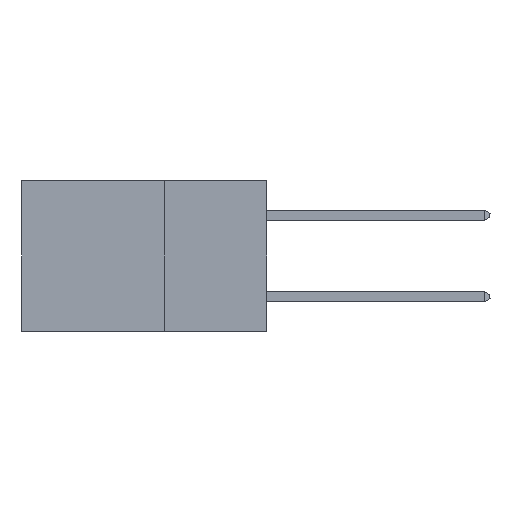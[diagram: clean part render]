
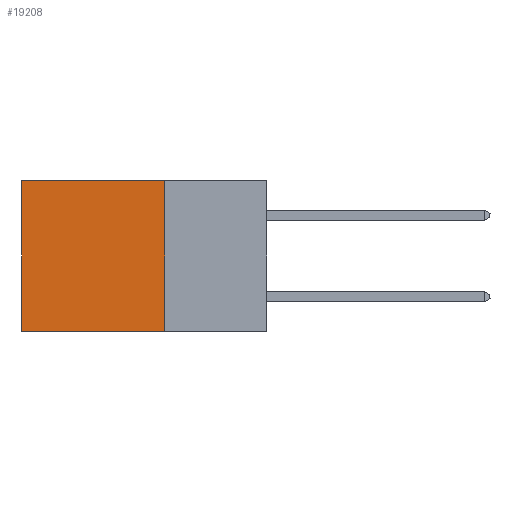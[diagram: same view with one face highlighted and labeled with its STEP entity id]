
A CAD part, left-side view. The second image highlights one B-rep face of the part: STEP entity #19208.
In plain terms, the highlighted planar face has unit normal (-1, 0, 0).
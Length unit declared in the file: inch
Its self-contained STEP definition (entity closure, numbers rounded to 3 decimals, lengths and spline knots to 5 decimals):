
#110 = LINE ( 'NONE', #9441, #12483 ) ;
#734 = VERTEX_POINT ( 'NONE', #19509 ) ;
#827 = CARTESIAN_POINT ( 'NONE',  ( 0.2875, 0.25, -0.37 ) ) ;
#2845 = CARTESIAN_POINT ( 'NONE',  ( 0.2875, 0.25, 0. ) ) ;
#3093 = LINE ( 'NONE', #20275, #16312 ) ;
#3643 = CARTESIAN_POINT ( 'NONE',  ( 0.2875, 0.6, 0. ) ) ;
#5081 = EDGE_CURVE ( 'NONE', #20559, #734, #110, .T. ) ;
#5331 = ORIENTED_EDGE ( 'NONE', *, *, #21031, .F. ) ;
#6045 = EDGE_LOOP ( 'NONE', ( #14767, #22066, #5331, #17293 ) ) ;
#6110 = VERTEX_POINT ( 'NONE', #827 ) ;
#8019 = CARTESIAN_POINT ( 'NONE',  ( 0.2875, 0.25, 0. ) ) ;
#8345 = VECTOR ( 'NONE', #12930, 39.37008 ) ;
#8389 = LINE ( 'NONE', #3643, #12555 ) ;
#8440 = CARTESIAN_POINT ( 'NONE',  ( 0.2875, 0.6, -0.37 ) ) ;
#8892 = LINE ( 'NONE', #11124, #8345 ) ;
#9387 = DIRECTION ( 'NONE',  ( 0., 1., 0. ) ) ;
#9441 = CARTESIAN_POINT ( 'NONE',  ( 0.2875, 0.25, 0. ) ) ;
#10845 = EDGE_CURVE ( 'NONE', #6110, #20611, #8892, .T. ) ;
#11124 = CARTESIAN_POINT ( 'NONE',  ( 0.2875, 0.25, -0.37 ) ) ;
#11577 = DIRECTION ( 'NONE',  ( 0., 0., -1. ) ) ;
#12483 = VECTOR ( 'NONE', #9387, 39.37008 ) ;
#12555 = VECTOR ( 'NONE', #12639, 39.37008 ) ;
#12639 = DIRECTION ( 'NONE',  ( 0., 0., -1. ) ) ;
#12930 = DIRECTION ( 'NONE',  ( 0., 1., 0. ) ) ;
#14767 = ORIENTED_EDGE ( 'NONE', *, *, #18281, .T. ) ;
#16312 = VECTOR ( 'NONE', #22013, 39.37008 ) ;
#17293 = ORIENTED_EDGE ( 'NONE', *, *, #5081, .T. ) ;
#17951 = AXIS2_PLACEMENT_3D ( 'NONE', #8019, #22224, #11577 ) ;
#18281 = EDGE_CURVE ( 'NONE', #734, #20611, #8389, .T. ) ;
#18712 = PLANE ( 'NONE',  #17951 ) ;
#19208 = ADVANCED_FACE ( 'NONE', ( #22758 ), #18712, .F. ) ;
#19509 = CARTESIAN_POINT ( 'NONE',  ( 0.2875, 0.6, 0. ) ) ;
#20275 = CARTESIAN_POINT ( 'NONE',  ( 0.2875, 0.25, 0. ) ) ;
#20559 = VERTEX_POINT ( 'NONE', #2845 ) ;
#20611 = VERTEX_POINT ( 'NONE', #8440 ) ;
#21031 = EDGE_CURVE ( 'NONE', #20559, #6110, #3093, .T. ) ;
#22013 = DIRECTION ( 'NONE',  ( 0., 0., -1. ) ) ;
#22066 = ORIENTED_EDGE ( 'NONE', *, *, #10845, .F. ) ;
#22224 = DIRECTION ( 'NONE',  ( 1., 0., 0. ) ) ;
#22758 = FACE_OUTER_BOUND ( 'NONE', #6045, .T. ) ;
